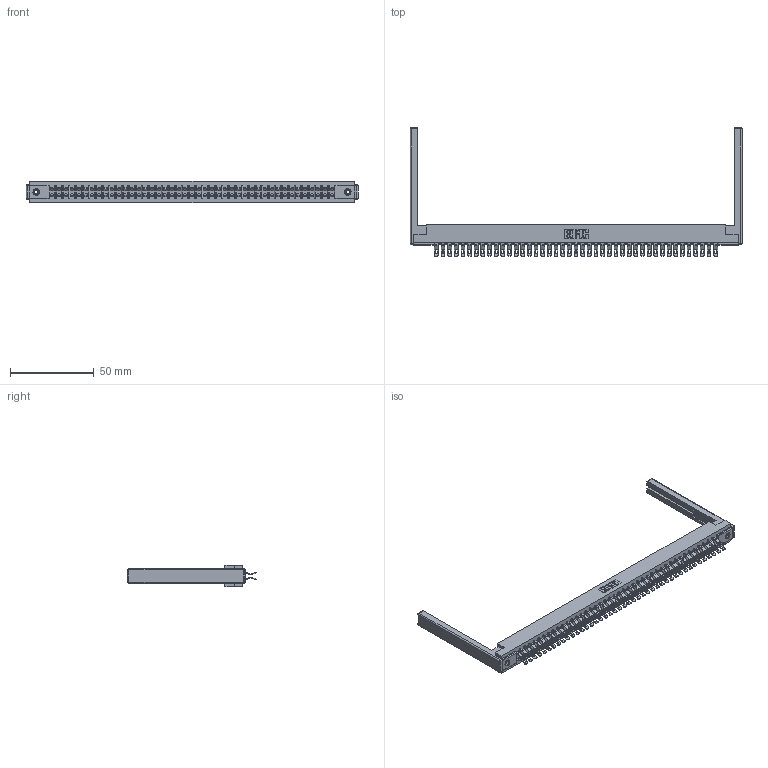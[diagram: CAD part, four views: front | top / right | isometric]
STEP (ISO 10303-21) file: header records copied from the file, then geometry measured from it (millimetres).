
FILE_DESCRIPTION (( 'STEP AP203' ), '1' );
FILE_NAME ('357-086-555-268.STEP', '2019-09-19T19:23:07', ( '' ), ( '' ), 'SwSTEP 2.0', 'SolidWorks 2016', '' );
FILE_SCHEMA (( 'CONFIG_CONTROL_DESIGN' ));
Length unit declared in the file: inch
Products named in the file (5): 307-220-068; 357-086-555-268; 307 Part_.156 Dia Mounting Holes; 345-250-001_345-250-001-102; 307-290-001_555
Assembly tree (91 placements, depth 2):
  357-086-555-268
    307 Part_.156 Dia Mounting Holes
    307-290-001_555  x86
    307-220-068  x2
    345-250-001_345-250-001-102  x2
Bounding box: 197.82 x 76.71 x 12.7 mm (x, y, z)
Volume: 25679.2 mm3; surface area: 31484.4 mm2
Topology: 91 solids, 91 shells, 5562 faces, 16279 edges, 10598 vertices
Faces by surface type: plane 3082, cylinder 2368, sphere 96, cone 12, torus 4
Entity records: 41412 total; most frequent: CARTESIAN_POINT 6756, ORIENTED_EDGE 6690, DIRECTION 6639, EDGE_CURVE 3345, VECTOR 2553, LINE 2553, VERTEX_POINT 2160, AXIS2_PLACEMENT_3D 2043
